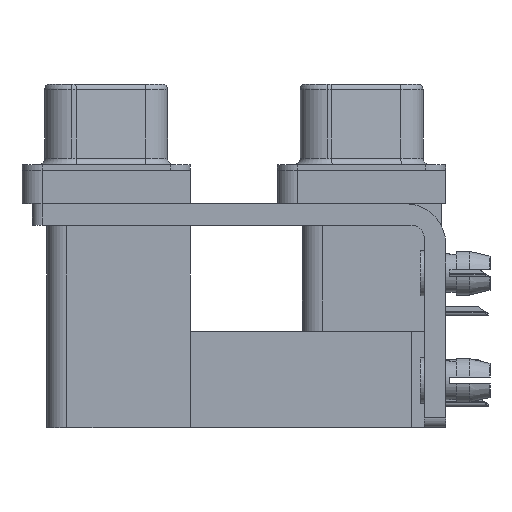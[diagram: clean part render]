
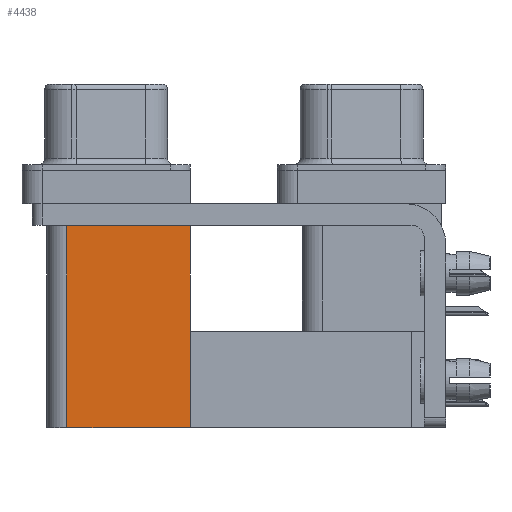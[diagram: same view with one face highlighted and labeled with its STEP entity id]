
A CAD part, left-side view. The second image highlights one B-rep face of the part: STEP entity #4438.
In plain terms, the highlighted planar face has unit normal (-1, 0, 0).
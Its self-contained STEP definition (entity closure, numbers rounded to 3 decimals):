
#3136 = AXIS2_PLACEMENT_3D ( 'NONE', #6967, #6389, #27477 ) ;
#3174 = CARTESIAN_POINT ( 'NONE',  ( 3.7, 12.775, -19.2 ) ) ;
#4135 = LINE ( 'NONE', #18257, #17247 ) ;
#4438 = ADVANCED_FACE ( 'NONE', ( #19015 ), #12596, .F. ) ;
#4720 = CARTESIAN_POINT ( 'NONE',  ( 3.7, 12.775, -19.2 ) ) ;
#4920 = DIRECTION ( 'NONE',  ( 0., 0., 1. ) ) ;
#5205 = VERTEX_POINT ( 'NONE', #8458 ) ;
#6389 = DIRECTION ( 'NONE',  ( 1., 0., 0. ) ) ;
#6967 = CARTESIAN_POINT ( 'NONE',  ( 3.7, 12.775, -19.2 ) ) ;
#7075 = EDGE_LOOP ( 'NONE', ( #32914, #19595, #31802, #38860 ) ) ;
#8458 = CARTESIAN_POINT ( 'NONE',  ( 3.7, 12.775, -2.5 ) ) ;
#8882 = VECTOR ( 'NONE', #4920, 1000. ) ;
#10339 = LINE ( 'NONE', #4720, #8882 ) ;
#11057 = VERTEX_POINT ( 'NONE', #3174 ) ;
#12596 = PLANE ( 'NONE',  #3136 ) ;
#14998 = CARTESIAN_POINT ( 'NONE',  ( 3.7, 12.775, -19.2 ) ) ;
#17247 = VECTOR ( 'NONE', #28044, 1000. ) ;
#17510 = VERTEX_POINT ( 'NONE', #30591 ) ;
#17801 = VERTEX_POINT ( 'NONE', #23515 ) ;
#18257 = CARTESIAN_POINT ( 'NONE',  ( 3.7, 12.775, -2.5 ) ) ;
#19015 = FACE_OUTER_BOUND ( 'NONE', #7075, .T. ) ;
#19595 = ORIENTED_EDGE ( 'NONE', *, *, #38391, .F. ) ;
#22764 = LINE ( 'NONE', #29206, #38223 ) ;
#23515 = CARTESIAN_POINT ( 'NONE',  ( 3.7, 21.975, -2.5 ) ) ;
#24040 = DIRECTION ( 'NONE',  ( 0., 1., 0. ) ) ;
#26707 = EDGE_CURVE ( 'NONE', #11057, #5205, #10339, .T. ) ;
#27477 = DIRECTION ( 'NONE',  ( 0., 1., 0. ) ) ;
#28044 = DIRECTION ( 'NONE',  ( 0., 1., 0. ) ) ;
#29031 = EDGE_CURVE ( 'NONE', #5205, #17801, #4135, .T. ) ;
#29206 = CARTESIAN_POINT ( 'NONE',  ( 3.7, 21.975, -19.2 ) ) ;
#29392 = DIRECTION ( 'NONE',  ( 0., 0., 1. ) ) ;
#30591 = CARTESIAN_POINT ( 'NONE',  ( 3.7, 21.975, -19.2 ) ) ;
#31469 = EDGE_CURVE ( 'NONE', #11057, #17510, #39505, .T. ) ;
#31481 = VECTOR ( 'NONE', #24040, 1000. ) ;
#31802 = ORIENTED_EDGE ( 'NONE', *, *, #31469, .F. ) ;
#32914 = ORIENTED_EDGE ( 'NONE', *, *, #29031, .T. ) ;
#38223 = VECTOR ( 'NONE', #29392, 1000. ) ;
#38391 = EDGE_CURVE ( 'NONE', #17510, #17801, #22764, .T. ) ;
#38860 = ORIENTED_EDGE ( 'NONE', *, *, #26707, .T. ) ;
#39505 = LINE ( 'NONE', #14998, #31481 ) ;
